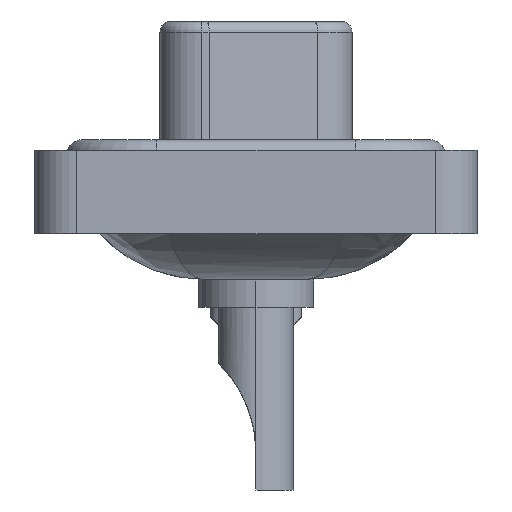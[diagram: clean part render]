
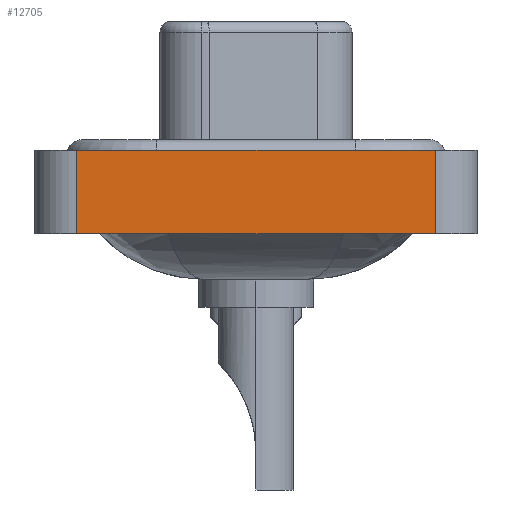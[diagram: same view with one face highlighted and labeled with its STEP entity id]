
A CAD part, left-side view. The second image highlights one B-rep face of the part: STEP entity #12705.
In plain terms, the highlighted planar face has unit normal (-1, 0, 0).
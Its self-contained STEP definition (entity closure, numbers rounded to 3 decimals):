
#533 = ORIENTED_EDGE ( 'NONE', *, *, #4223, .F. ) ;
#595 = EDGE_LOOP ( 'NONE', ( #6740, #533, #21735, #4452 ) ) ;
#813 = LINE ( 'NONE', #4616, #16475 ) ;
#1154 = CARTESIAN_POINT ( 'NONE',  ( -7.35, -8.55, -3.6 ) ) ;
#3095 = DIRECTION ( 'NONE',  ( 0., -1., 0. ) ) ;
#4223 = EDGE_CURVE ( 'NONE', #21510, #5293, #11661, .T. ) ;
#4366 = VECTOR ( 'NONE', #3095, 1000. ) ;
#4452 = ORIENTED_EDGE ( 'NONE', *, *, #12589, .T. ) ;
#4616 = CARTESIAN_POINT ( 'NONE',  ( -7.35, -8.55, -3.6 ) ) ;
#5293 = VERTEX_POINT ( 'NONE', #6571 ) ;
#6571 = CARTESIAN_POINT ( 'NONE',  ( -7.35, -8.55, 0.4 ) ) ;
#6740 = ORIENTED_EDGE ( 'NONE', *, *, #21651, .T. ) ;
#7418 = LINE ( 'NONE', #15544, #21942 ) ;
#8837 = LINE ( 'NONE', #19263, #12421 ) ;
#8940 = CARTESIAN_POINT ( 'NONE',  ( -7.35, 8.55, -3.6 ) ) ;
#8944 = DIRECTION ( 'NONE',  ( 0., 0., 1. ) ) ;
#9696 = FACE_OUTER_BOUND ( 'NONE', #595, .T. ) ;
#11661 = LINE ( 'NONE', #18476, #4366 ) ;
#12421 = VECTOR ( 'NONE', #8944, 1000. ) ;
#12589 = EDGE_CURVE ( 'NONE', #17412, #12690, #813, .T. ) ;
#12690 = VERTEX_POINT ( 'NONE', #18217 ) ;
#12705 = ADVANCED_FACE ( 'NONE', ( #9696 ), #16554, .T. ) ;
#14179 = DIRECTION ( 'NONE',  ( 0., 0., 1. ) ) ;
#14869 = DIRECTION ( 'NONE',  ( -1., 0., 0. ) ) ;
#15544 = CARTESIAN_POINT ( 'NONE',  ( -7.35, -8.55, -3.6 ) ) ;
#16444 = DIRECTION ( 'NONE',  ( 0., -1., 0. ) ) ;
#16475 = VECTOR ( 'NONE', #16444, 1000. ) ;
#16554 = PLANE ( 'NONE',  #20749 ) ;
#17310 = CARTESIAN_POINT ( 'NONE',  ( -7.35, 8.55, 0.4 ) ) ;
#17412 = VERTEX_POINT ( 'NONE', #8940 ) ;
#18217 = CARTESIAN_POINT ( 'NONE',  ( -7.35, -8.55, -3.6 ) ) ;
#18476 = CARTESIAN_POINT ( 'NONE',  ( -7.35, -8.55, 0.4 ) ) ;
#18885 = EDGE_CURVE ( 'NONE', #17412, #21510, #8837, .T. ) ;
#19263 = CARTESIAN_POINT ( 'NONE',  ( -7.35, 8.55, -3.6 ) ) ;
#20749 = AXIS2_PLACEMENT_3D ( 'NONE', #1154, #14869, #21685 ) ;
#21510 = VERTEX_POINT ( 'NONE', #17310 ) ;
#21651 = EDGE_CURVE ( 'NONE', #12690, #5293, #7418, .T. ) ;
#21685 = DIRECTION ( 'NONE',  ( 0., 0., 1. ) ) ;
#21735 = ORIENTED_EDGE ( 'NONE', *, *, #18885, .F. ) ;
#21942 = VECTOR ( 'NONE', #14179, 1000. ) ;
